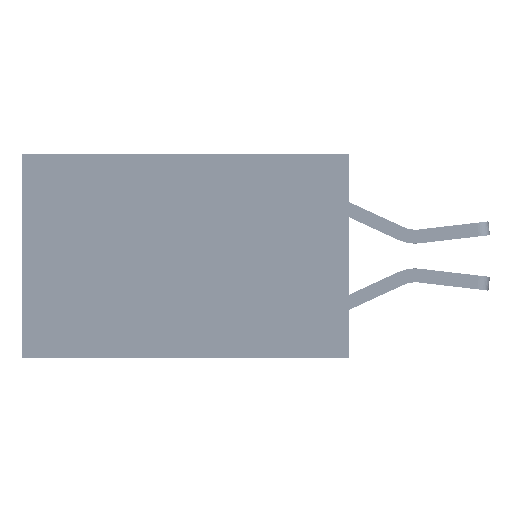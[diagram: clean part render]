
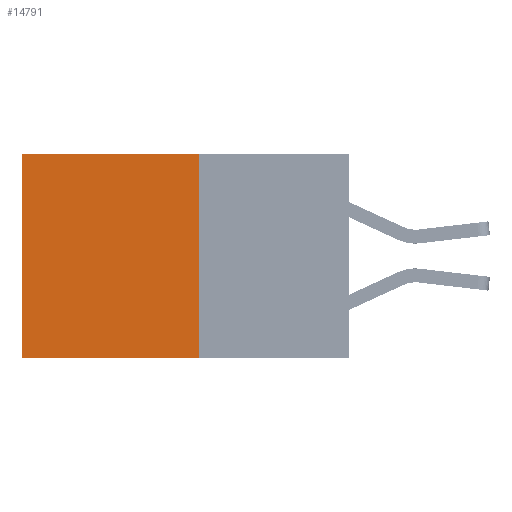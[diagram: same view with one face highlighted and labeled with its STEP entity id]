
A CAD part, left-side view. The second image highlights one B-rep face of the part: STEP entity #14791.
In plain terms, the highlighted planar face has unit normal (-1, 0, 0).
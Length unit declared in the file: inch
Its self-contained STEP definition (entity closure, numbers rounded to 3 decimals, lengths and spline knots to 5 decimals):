
#200 = VECTOR ( 'NONE', #13285, 39.37008 ) ;
#622 = ORIENTED_EDGE ( 'NONE', *, *, #12932, .F. ) ;
#1193 = LINE ( 'NONE', #26848, #28703 ) ;
#1967 = CARTESIAN_POINT ( 'NONE',  ( 0.277, 0.59, -0.37 ) ) ;
#2035 = PLANE ( 'NONE',  #19791 ) ;
#2610 = CARTESIAN_POINT ( 'NONE',  ( 0.277, 0.27, -0.37 ) ) ;
#3648 = CARTESIAN_POINT ( 'NONE',  ( 0.277, 0.27, 0. ) ) ;
#3711 = CARTESIAN_POINT ( 'NONE',  ( 0.277, 0.27, 0. ) ) ;
#4380 = LINE ( 'NONE', #11751, #18293 ) ;
#6859 = FACE_OUTER_BOUND ( 'NONE', #20908, .T. ) ;
#7355 = LINE ( 'NONE', #2610, #200 ) ;
#7453 = DIRECTION ( 'NONE',  ( 1., 0., 0. ) ) ;
#9345 = CARTESIAN_POINT ( 'NONE',  ( 0.277, 0.27, -0.37 ) ) ;
#10514 = VERTEX_POINT ( 'NONE', #9345 ) ;
#11600 = DIRECTION ( 'NONE',  ( 0., 0., -1. ) ) ;
#11751 = CARTESIAN_POINT ( 'NONE',  ( 0.277, 0.27, -0.37 ) ) ;
#12932 = EDGE_CURVE ( 'NONE', #10514, #14127, #7355, .T. ) ;
#13284 = EDGE_CURVE ( 'NONE', #28395, #10514, #4380, .T. ) ;
#13285 = DIRECTION ( 'NONE',  ( 0., 1., 0. ) ) ;
#14127 = VERTEX_POINT ( 'NONE', #1967 ) ;
#14659 = ORIENTED_EDGE ( 'NONE', *, *, #26991, .T. ) ;
#14791 = ADVANCED_FACE ( 'NONE', ( #6859 ), #2035, .F. ) ;
#15012 = CARTESIAN_POINT ( 'NONE',  ( 0.277, 0.59, 0. ) ) ;
#15240 = CARTESIAN_POINT ( 'NONE',  ( 0.277, 0.27, -0.37 ) ) ;
#15510 = VERTEX_POINT ( 'NONE', #15012 ) ;
#18293 = VECTOR ( 'NONE', #19536, 39.37008 ) ;
#18809 = LINE ( 'NONE', #3711, #25526 ) ;
#19536 = DIRECTION ( 'NONE',  ( 0., 0., -1. ) ) ;
#19791 = AXIS2_PLACEMENT_3D ( 'NONE', #15240, #7453, #25418 ) ;
#20908 = EDGE_LOOP ( 'NONE', ( #23263, #622, #26694, #14659 ) ) ;
#21916 = DIRECTION ( 'NONE',  ( 0., 1., 0. ) ) ;
#23263 = ORIENTED_EDGE ( 'NONE', *, *, #31609, .T. ) ;
#25418 = DIRECTION ( 'NONE',  ( 0., 0., -1. ) ) ;
#25526 = VECTOR ( 'NONE', #21916, 39.37008 ) ;
#26694 = ORIENTED_EDGE ( 'NONE', *, *, #13284, .F. ) ;
#26848 = CARTESIAN_POINT ( 'NONE',  ( 0.277, 0.59, -0.37 ) ) ;
#26991 = EDGE_CURVE ( 'NONE', #28395, #15510, #18809, .T. ) ;
#28395 = VERTEX_POINT ( 'NONE', #3648 ) ;
#28703 = VECTOR ( 'NONE', #11600, 39.37008 ) ;
#31609 = EDGE_CURVE ( 'NONE', #15510, #14127, #1193, .T. ) ;
